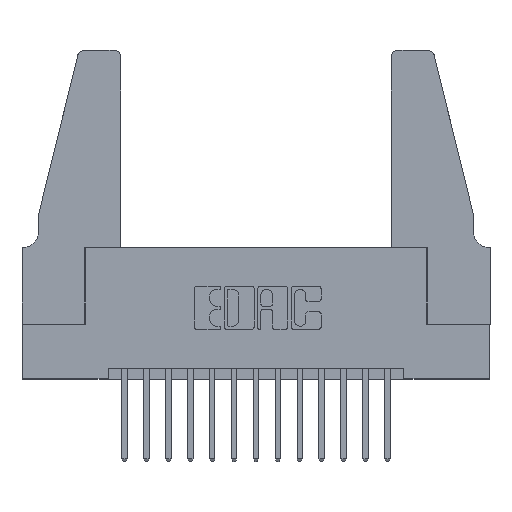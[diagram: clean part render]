
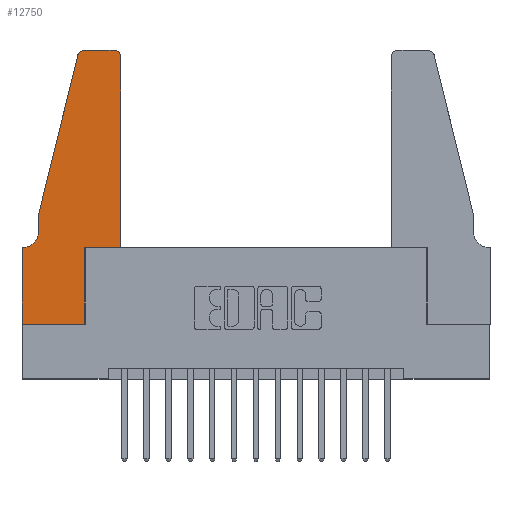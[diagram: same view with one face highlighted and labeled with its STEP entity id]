
A CAD part, top view. The second image highlights one B-rep face of the part: STEP entity #12750.
In plain terms, the highlighted planar face has unit normal (0, 0, 1).
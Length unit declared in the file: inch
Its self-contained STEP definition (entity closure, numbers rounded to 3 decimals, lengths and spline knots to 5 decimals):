
#159 = DIRECTION ( 'NONE',  ( 0., 0., 1. ) ) ;
#181 = CARTESIAN_POINT ( 'NONE',  ( 0.25487, 1.22718, 0.37 ) ) ;
#242 = DIRECTION ( 'NONE',  ( 1., 0., 0. ) ) ;
#354 = ORIENTED_EDGE ( 'NONE', *, *, #1998, .T. ) ;
#784 = ORIENTED_EDGE ( 'NONE', *, *, #5137, .T. ) ;
#1126 = CARTESIAN_POINT ( 'NONE',  ( 0., 0.35, 0.37 ) ) ;
#1282 = VERTEX_POINT ( 'NONE', #4204 ) ;
#1490 = DIRECTION ( 'NONE',  ( -1., 0., 0. ) ) ;
#1649 = EDGE_CURVE ( 'NONE', #11172, #14732, #12398, .T. ) ;
#1955 = VECTOR ( 'NONE', #5379, 39.37008 ) ;
#1983 = ORIENTED_EDGE ( 'NONE', *, *, #1649, .T. ) ;
#1998 = EDGE_CURVE ( 'NONE', #11078, #3709, #12795, .T. ) ;
#2039 = LINE ( 'NONE', #8408, #5785 ) ;
#2395 = CARTESIAN_POINT ( 'NONE',  ( 0.0755, 0.5, 0.37 ) ) ;
#2559 = LINE ( 'NONE', #2395, #5522 ) ;
#2641 = DIRECTION ( 'NONE',  ( 0., -1., 0. ) ) ;
#2735 = EDGE_LOOP ( 'NONE', ( #13948, #354, #5108, #7766, #13350, #6585, #7649, #7436, #15369, #1983, #784, #4957 ) ) ;
#3649 = EDGE_CURVE ( 'NONE', #3709, #14912, #2559, .T. ) ;
#3709 = VERTEX_POINT ( 'NONE', #181 ) ;
#4004 = CARTESIAN_POINT ( 'NONE',  ( 0.2865, 0.35, 0.37 ) ) ;
#4036 = AXIS2_PLACEMENT_3D ( 'NONE', #10181, #12666, #9350 ) ;
#4083 = AXIS2_PLACEMENT_3D ( 'NONE', #15668, #11914, #6752 ) ;
#4204 = CARTESIAN_POINT ( 'NONE',  ( 0.0055, 0.35, 0.37 ) ) ;
#4749 = VERTEX_POINT ( 'NONE', #9691 ) ;
#4957 = ORIENTED_EDGE ( 'NONE', *, *, #14146, .T. ) ;
#4975 = VECTOR ( 'NONE', #2641, 39.37008 ) ;
#4982 = DIRECTION ( 'NONE',  ( 1., 0., 0. ) ) ;
#5108 = ORIENTED_EDGE ( 'NONE', *, *, #3649, .T. ) ;
#5109 = CARTESIAN_POINT ( 'NONE',  ( 0.0755, 0.35, 0.37 ) ) ;
#5137 = EDGE_CURVE ( 'NONE', #14732, #12718, #8588, .T. ) ;
#5279 = EDGE_CURVE ( 'NONE', #9710, #11172, #8775, .T. ) ;
#5281 = CIRCLE ( 'NONE', #4036, 0.07 ) ;
#5379 = DIRECTION ( 'NONE',  ( 0., 1., 0. ) ) ;
#5522 = VECTOR ( 'NONE', #6137, 39.37008 ) ;
#5598 = LINE ( 'NONE', #11304, #9097 ) ;
#5785 = VECTOR ( 'NONE', #12172, 39.37008 ) ;
#5933 = AXIS2_PLACEMENT_3D ( 'NONE', #15237, #159, #10223 ) ;
#6087 = LINE ( 'NONE', #5109, #7835 ) ;
#6137 = DIRECTION ( 'NONE',  ( -0.239, -0.971, 0. ) ) ;
#6585 = ORIENTED_EDGE ( 'NONE', *, *, #15712, .T. ) ;
#6752 = DIRECTION ( 'NONE',  ( 1., 0., 0. ) ) ;
#6833 = EDGE_CURVE ( 'NONE', #7830, #9710, #5598, .T. ) ;
#7140 = CARTESIAN_POINT ( 'NONE',  ( 0., 0., 0.37 ) ) ;
#7242 = CARTESIAN_POINT ( 'NONE',  ( 0.0755, 0.5, 0.37 ) ) ;
#7294 = EDGE_CURVE ( 'NONE', #10140, #11078, #2039, .T. ) ;
#7436 = ORIENTED_EDGE ( 'NONE', *, *, #6833, .T. ) ;
#7452 = VERTEX_POINT ( 'NONE', #13402 ) ;
#7486 = DIRECTION ( 'NONE',  ( 0., 0., 1. ) ) ;
#7649 = ORIENTED_EDGE ( 'NONE', *, *, #14749, .T. ) ;
#7766 = ORIENTED_EDGE ( 'NONE', *, *, #13417, .T. ) ;
#7830 = VERTEX_POINT ( 'NONE', #11491 ) ;
#7835 = VECTOR ( 'NONE', #1490, 39.37008 ) ;
#8061 = CARTESIAN_POINT ( 'NONE',  ( 0.2865, 0.35, 0.37 ) ) ;
#8408 = CARTESIAN_POINT ( 'NONE',  ( 0.2605, 1.25, 0.37 ) ) ;
#8588 = LINE ( 'NONE', #15355, #14536 ) ;
#8664 = LINE ( 'NONE', #14890, #4975 ) ;
#8695 = VECTOR ( 'NONE', #15709, 39.37008 ) ;
#8775 = LINE ( 'NONE', #4004, #1955 ) ;
#9024 = CARTESIAN_POINT ( 'NONE',  ( 0.4205, 1.25, 0.37 ) ) ;
#9048 = CARTESIAN_POINT ( 'NONE',  ( 0.4505, 0.35, 0.37 ) ) ;
#9097 = VECTOR ( 'NONE', #242, 39.37008 ) ;
#9350 = DIRECTION ( 'NONE',  ( -1., 0., 0. ) ) ;
#9481 = CARTESIAN_POINT ( 'NONE',  ( 0.4505, 0.35, 0.37 ) ) ;
#9691 = CARTESIAN_POINT ( 'NONE',  ( 0.0755, 0.42, 0.37 ) ) ;
#9710 = VERTEX_POINT ( 'NONE', #12276 ) ;
#9853 = VECTOR ( 'NONE', #13458, 39.37008 ) ;
#9862 = EDGE_CURVE ( 'NONE', #4749, #1282, #5281, .T. ) ;
#9910 = FACE_OUTER_BOUND ( 'NONE', #2735, .T. ) ;
#10140 = VERTEX_POINT ( 'NONE', #9024 ) ;
#10181 = CARTESIAN_POINT ( 'NONE',  ( 0.0055, 0.42, 0.37 ) ) ;
#10223 = DIRECTION ( 'NONE',  ( 1., 0., 0. ) ) ;
#10647 = CIRCLE ( 'NONE', #4083, 0.03 ) ;
#11011 = LINE ( 'NONE', #7140, #9853 ) ;
#11078 = VERTEX_POINT ( 'NONE', #11922 ) ;
#11172 = VERTEX_POINT ( 'NONE', #8061 ) ;
#11304 = CARTESIAN_POINT ( 'NONE',  ( 0., 0., 0.37 ) ) ;
#11491 = CARTESIAN_POINT ( 'NONE',  ( 0., 0., 0.37 ) ) ;
#11914 = DIRECTION ( 'NONE',  ( 0., 0., 1. ) ) ;
#11922 = CARTESIAN_POINT ( 'NONE',  ( 0.284, 1.25, 0.37 ) ) ;
#12172 = DIRECTION ( 'NONE',  ( -1., 0., 0. ) ) ;
#12276 = CARTESIAN_POINT ( 'NONE',  ( 0.2865, 0., 0.37 ) ) ;
#12398 = LINE ( 'NONE', #9481, #8695 ) ;
#12666 = DIRECTION ( 'NONE',  ( 0., 0., -1. ) ) ;
#12718 = VERTEX_POINT ( 'NONE', #14913 ) ;
#12750 = ADVANCED_FACE ( 'NONE', ( #9910 ), #15031, .T. ) ;
#12795 = CIRCLE ( 'NONE', #5933, 0.03 ) ;
#13350 = ORIENTED_EDGE ( 'NONE', *, *, #9862, .T. ) ;
#13402 = CARTESIAN_POINT ( 'NONE',  ( 0., 0.35, 0.37 ) ) ;
#13417 = EDGE_CURVE ( 'NONE', #14912, #4749, #8664, .T. ) ;
#13458 = DIRECTION ( 'NONE',  ( 0., -1., 0. ) ) ;
#13948 = ORIENTED_EDGE ( 'NONE', *, *, #7294, .T. ) ;
#14146 = EDGE_CURVE ( 'NONE', #12718, #10140, #10647, .T. ) ;
#14523 = DIRECTION ( 'NONE',  ( 0., 1., 0. ) ) ;
#14536 = VECTOR ( 'NONE', #14523, 39.37008 ) ;
#14732 = VERTEX_POINT ( 'NONE', #9048 ) ;
#14749 = EDGE_CURVE ( 'NONE', #7452, #7830, #11011, .T. ) ;
#14890 = CARTESIAN_POINT ( 'NONE',  ( 0.0755, 0.5, 0.37 ) ) ;
#14912 = VERTEX_POINT ( 'NONE', #7242 ) ;
#14913 = CARTESIAN_POINT ( 'NONE',  ( 0.4505, 1.22, 0.37 ) ) ;
#15031 = PLANE ( 'NONE',  #15971 ) ;
#15237 = CARTESIAN_POINT ( 'NONE',  ( 0.284, 1.22, 0.37 ) ) ;
#15355 = CARTESIAN_POINT ( 'NONE',  ( 0.4505, 0.35, 0.37 ) ) ;
#15369 = ORIENTED_EDGE ( 'NONE', *, *, #5279, .T. ) ;
#15668 = CARTESIAN_POINT ( 'NONE',  ( 0.4205, 1.22, 0.37 ) ) ;
#15709 = DIRECTION ( 'NONE',  ( 1., 0., 0. ) ) ;
#15712 = EDGE_CURVE ( 'NONE', #1282, #7452, #6087, .T. ) ;
#15971 = AXIS2_PLACEMENT_3D ( 'NONE', #1126, #7486, #4982 ) ;
